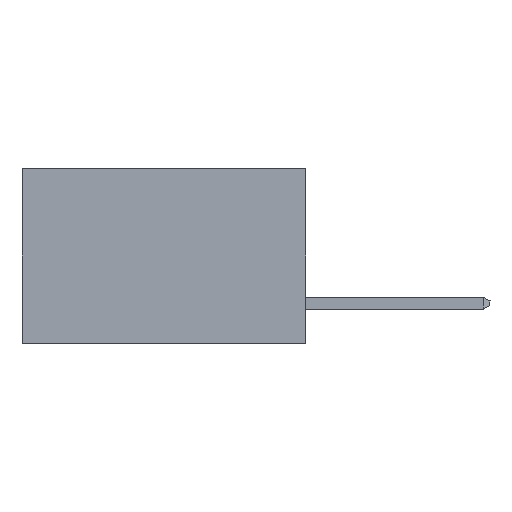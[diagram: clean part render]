
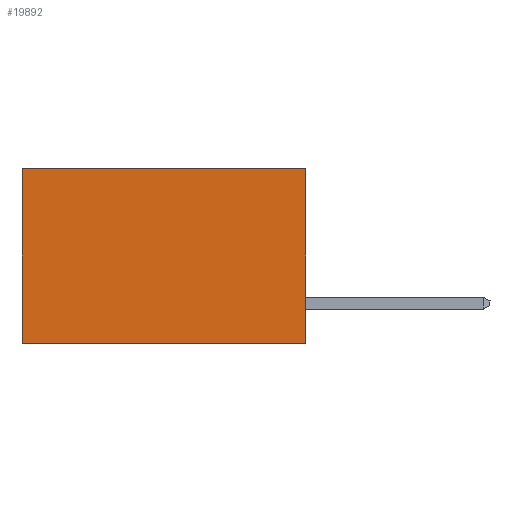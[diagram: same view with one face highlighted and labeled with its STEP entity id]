
A CAD part, left-side view. The second image highlights one B-rep face of the part: STEP entity #19892.
In plain terms, the highlighted planar face has unit normal (-1, 0, 0).
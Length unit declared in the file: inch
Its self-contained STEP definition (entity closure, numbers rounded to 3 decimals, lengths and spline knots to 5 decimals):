
#844 = DIRECTION ( 'NONE',  ( 0., 1., 0. ) ) ;
#858 = ORIENTED_EDGE ( 'NONE', *, *, #16262, .T. ) ;
#1348 = DIRECTION ( 'NONE',  ( 1., 0., 0. ) ) ;
#1429 = CARTESIAN_POINT ( 'NONE',  ( 0.298, 0., 0. ) ) ;
#3518 = LINE ( 'NONE', #9476, #15224 ) ;
#4828 = DIRECTION ( 'NONE',  ( 0., 0., -1. ) ) ;
#5022 = EDGE_CURVE ( 'NONE', #8440, #17661, #5730, .T. ) ;
#5048 = VERTEX_POINT ( 'NONE', #21868 ) ;
#5312 = EDGE_CURVE ( 'NONE', #5048, #8440, #23676, .T. ) ;
#5544 = CARTESIAN_POINT ( 'NONE',  ( 0.298, 0., 0. ) ) ;
#5730 = LINE ( 'NONE', #16125, #12952 ) ;
#7173 = DIRECTION ( 'NONE',  ( 0., 0., -1. ) ) ;
#8169 = CARTESIAN_POINT ( 'NONE',  ( 0.298, 0., 0. ) ) ;
#8423 = VECTOR ( 'NONE', #4828, 39.37008 ) ;
#8440 = VERTEX_POINT ( 'NONE', #15688 ) ;
#8560 = ORIENTED_EDGE ( 'NONE', *, *, #5312, .F. ) ;
#9345 = ORIENTED_EDGE ( 'NONE', *, *, #21748, .T. ) ;
#9476 = CARTESIAN_POINT ( 'NONE',  ( 0.298, 0.6, 0. ) ) ;
#9782 = VERTEX_POINT ( 'NONE', #20130 ) ;
#10793 = ORIENTED_EDGE ( 'NONE', *, *, #5022, .F. ) ;
#12952 = VECTOR ( 'NONE', #844, 39.37008 ) ;
#12971 = PLANE ( 'NONE',  #15317 ) ;
#13326 = DIRECTION ( 'NONE',  ( 0., 0., -1. ) ) ;
#14176 = CARTESIAN_POINT ( 'NONE',  ( 0.298, 0.6, -0.37 ) ) ;
#14813 = EDGE_LOOP ( 'NONE', ( #9345, #10793, #8560, #858 ) ) ;
#15224 = VECTOR ( 'NONE', #13326, 39.37008 ) ;
#15317 = AXIS2_PLACEMENT_3D ( 'NONE', #1429, #1348, #7173 ) ;
#15688 = CARTESIAN_POINT ( 'NONE',  ( 0.298, 0., -0.37 ) ) ;
#16125 = CARTESIAN_POINT ( 'NONE',  ( 0.298, 0., -0.37 ) ) ;
#16262 = EDGE_CURVE ( 'NONE', #5048, #9782, #20454, .T. ) ;
#17661 = VERTEX_POINT ( 'NONE', #14176 ) ;
#19892 = ADVANCED_FACE ( 'NONE', ( #23255 ), #12971, .F. ) ;
#20130 = CARTESIAN_POINT ( 'NONE',  ( 0.298, 0.6, 0. ) ) ;
#20139 = VECTOR ( 'NONE', #20716, 39.37008 ) ;
#20454 = LINE ( 'NONE', #5544, #20139 ) ;
#20716 = DIRECTION ( 'NONE',  ( 0., 1., 0. ) ) ;
#21748 = EDGE_CURVE ( 'NONE', #9782, #17661, #3518, .T. ) ;
#21868 = CARTESIAN_POINT ( 'NONE',  ( 0.298, 0., 0. ) ) ;
#23255 = FACE_OUTER_BOUND ( 'NONE', #14813, .T. ) ;
#23676 = LINE ( 'NONE', #8169, #8423 ) ;
